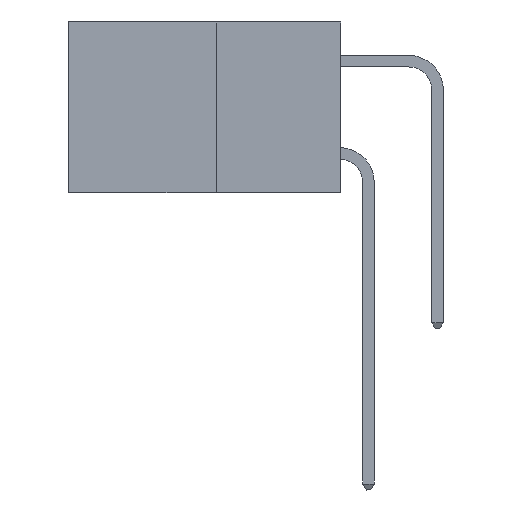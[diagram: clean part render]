
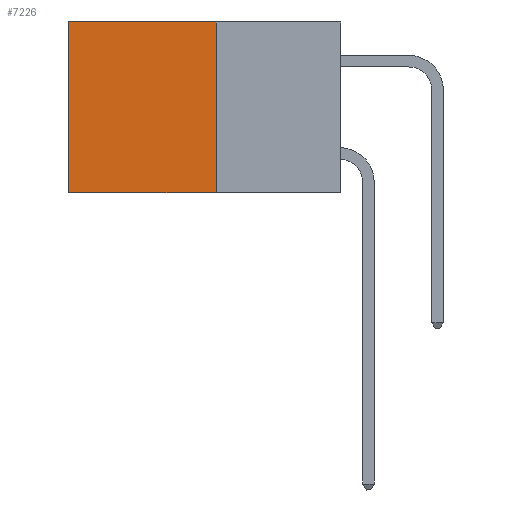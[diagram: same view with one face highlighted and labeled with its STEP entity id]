
A CAD part, left-side view. The second image highlights one B-rep face of the part: STEP entity #7226.
In plain terms, the highlighted planar face has unit normal (-1, 0, 0).
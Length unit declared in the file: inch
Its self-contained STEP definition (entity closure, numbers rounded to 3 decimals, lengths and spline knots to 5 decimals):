
#1501 = EDGE_CURVE ( 'NONE', #5988, #22129, #12081, .T. ) ;
#2918 = DIRECTION ( 'NONE',  ( 0., 1., 0. ) ) ;
#3562 = PLANE ( 'NONE',  #12618 ) ;
#3620 = CARTESIAN_POINT ( 'NONE',  ( 0.277, 0.27, 0. ) ) ;
#5760 = DIRECTION ( 'NONE',  ( 0., 0., -1. ) ) ;
#5932 = DIRECTION ( 'NONE',  ( 0., 1., 0. ) ) ;
#5988 = VERTEX_POINT ( 'NONE', #3620 ) ;
#6412 = DIRECTION ( 'NONE',  ( 0., 0., -1. ) ) ;
#7226 = ADVANCED_FACE ( 'NONE', ( #17363 ), #3562, .F. ) ;
#9254 = EDGE_CURVE ( 'NONE', #27083, #15580, #12913, .T. ) ;
#10122 = LINE ( 'NONE', #13729, #21526 ) ;
#10762 = ORIENTED_EDGE ( 'NONE', *, *, #9254, .T. ) ;
#11558 = EDGE_CURVE ( 'NONE', #5988, #27083, #10122, .T. ) ;
#12081 = LINE ( 'NONE', #15986, #23423 ) ;
#12115 = CARTESIAN_POINT ( 'NONE',  ( 0.277, 0.27, -0.37 ) ) ;
#12286 = CARTESIAN_POINT ( 'NONE',  ( 0.277, 0.27, -0.37 ) ) ;
#12618 = AXIS2_PLACEMENT_3D ( 'NONE', #12115, #18602, #5760 ) ;
#12913 = LINE ( 'NONE', #17119, #22914 ) ;
#13729 = CARTESIAN_POINT ( 'NONE',  ( 0.277, 0.27, 0. ) ) ;
#14981 = EDGE_LOOP ( 'NONE', ( #10762, #21083, #18029, #16991 ) ) ;
#15200 = CARTESIAN_POINT ( 'NONE',  ( 0.277, 0.27, -0.37 ) ) ;
#15580 = VERTEX_POINT ( 'NONE', #19175 ) ;
#15986 = CARTESIAN_POINT ( 'NONE',  ( 0.277, 0.27, -0.37 ) ) ;
#16381 = DIRECTION ( 'NONE',  ( 0., 0., -1. ) ) ;
#16654 = VECTOR ( 'NONE', #5932, 39.37008 ) ;
#16991 = ORIENTED_EDGE ( 'NONE', *, *, #11558, .T. ) ;
#17119 = CARTESIAN_POINT ( 'NONE',  ( 0.277, 0.59, -0.37 ) ) ;
#17328 = LINE ( 'NONE', #12286, #16654 ) ;
#17363 = FACE_OUTER_BOUND ( 'NONE', #14981, .T. ) ;
#18029 = ORIENTED_EDGE ( 'NONE', *, *, #1501, .F. ) ;
#18602 = DIRECTION ( 'NONE',  ( 1., 0., 0. ) ) ;
#19175 = CARTESIAN_POINT ( 'NONE',  ( 0.277, 0.59, -0.37 ) ) ;
#21083 = ORIENTED_EDGE ( 'NONE', *, *, #23254, .F. ) ;
#21526 = VECTOR ( 'NONE', #2918, 39.37008 ) ;
#22129 = VERTEX_POINT ( 'NONE', #15200 ) ;
#22708 = CARTESIAN_POINT ( 'NONE',  ( 0.277, 0.59, 0. ) ) ;
#22914 = VECTOR ( 'NONE', #6412, 39.37008 ) ;
#23254 = EDGE_CURVE ( 'NONE', #22129, #15580, #17328, .T. ) ;
#23423 = VECTOR ( 'NONE', #16381, 39.37008 ) ;
#27083 = VERTEX_POINT ( 'NONE', #22708 ) ;
